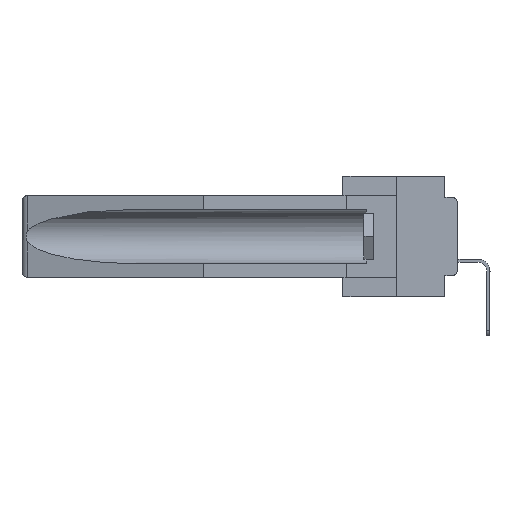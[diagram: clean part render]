
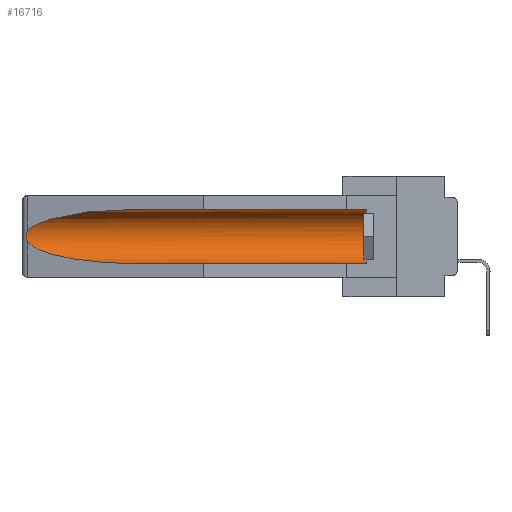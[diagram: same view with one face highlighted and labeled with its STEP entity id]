
A CAD part, left-side view. The second image highlights one B-rep face of the part: STEP entity #16716.
In plain terms, the highlighted cylindrical face has radius 2.857 mm (diameter 5.715 mm), a partial arc.
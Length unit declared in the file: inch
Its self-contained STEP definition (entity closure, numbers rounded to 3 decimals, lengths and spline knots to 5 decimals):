
#105 = CARTESIAN_POINT ( 'NONE',  ( 0.155, -0.30754, -0.059 ) ) ;
#718 = CARTESIAN_POINT ( 'NONE',  ( 0.26537, 1.52718, -0.14972 ) ) ;
#1028 = CARTESIAN_POINT ( 'NONE',  ( 0.155, -0.30754, -0.1715 ) ) ;
#1640 = ORIENTED_EDGE ( 'NONE', *, *, #16192, .T. ) ;
#2006 = CARTESIAN_POINT ( 'NONE',  ( 0.155, 1.07973, -0.059 ) ) ;
#2267 = CARTESIAN_POINT ( 'NONE',  ( 0.155, 1.07973, -0.284 ) ) ;
#2956 = VERTEX_POINT ( 'NONE', #7251 ) ;
#3813 = VERTEX_POINT ( 'NONE', #2006 ) ;
#4181 = CARTESIAN_POINT ( 'NONE',  ( 0.155, 0.126, -0.059 ) ) ;
#4958 = CARTESIAN_POINT ( 'NONE',  ( 0.26654, 1.53092, -0.15636 ) ) ;
#5268 = EDGE_LOOP ( 'NONE', ( #12434, #22318, #27496, #17590, #1640, #22767 ) ) ;
#5561 = CYLINDRICAL_SURFACE ( 'NONE', #6483, 0.1125 ) ;
#6483 = AXIS2_PLACEMENT_3D ( 'NONE', #1028, #25777, #22662 ) ;
#7251 = CARTESIAN_POINT ( 'NONE',  ( 0.26537, 1.52718, -0.19328 ) ) ;
#7701 = CARTESIAN_POINT ( 'NONE',  ( 0.2675, 1.53308, -0.17534 ) ) ;
#8160 = B_SPLINE_CURVE_WITH_KNOTS ( 'NONE', 3,
 ( #27314, #27443, #4958, #19149, #24191, #7701, #13264, #26968, #32794, #10482 ),
 .UNSPECIFIED., .F., .F.,
 ( 4, 2, 2, 2, 4 ),
 ( 0., 0.00029, 0.00058, 0.00087, 0.00117 ),
 .UNSPECIFIED. ) ;
#8380 = VERTEX_POINT ( 'NONE', #17113 ) ;
#10026 = VERTEX_POINT ( 'NONE', #23471 ) ;
#10482 = CARTESIAN_POINT ( 'NONE',  ( 0.26537, 1.52718, -0.19328 ) ) ;
#10791 = EDGE_CURVE ( 'NONE', #2956, #8380, #33728, .T. ) ;
#12370 = DIRECTION ( 'NONE',  ( 0., -1., 0. ) ) ;
#12434 = ORIENTED_EDGE ( 'NONE', *, *, #25221, .T. ) ;
#12537 = VECTOR ( 'NONE', #16839, 39.37008 ) ;
#13201 = CARTESIAN_POINT ( 'NONE',  ( 0.21114, 1.30732, -0.284 ) ) ;
#13264 = CARTESIAN_POINT ( 'NONE',  ( 0.2673, 1.53269, -0.17917 ) ) ;
#13552 = CARTESIAN_POINT ( 'NONE',  ( 0.26537, 1.52718, -0.19328 ) ) ;
#15893 = EDGE_CURVE ( 'NONE', #18064, #3813, #24154, .T. ) ;
#15982 = CARTESIAN_POINT ( 'NONE',  ( 0.155, -0.30754, -0.284 ) ) ;
#16192 = EDGE_CURVE ( 'NONE', #10026, #18064, #18959, .T. ) ;
#16415 = LINE ( 'NONE', #15982, #34472 ) ;
#16716 = ADVANCED_FACE ( 'NONE', ( #32641 ), #5561, .F. ) ;
#16839 = DIRECTION ( 'NONE',  ( 0., 1., 0. ) ) ;
#17113 = CARTESIAN_POINT ( 'NONE',  ( 0.155, 1.07973, -0.284 ) ) ;
#17590 = ORIENTED_EDGE ( 'NONE', *, *, #20968, .F. ) ;
#18064 = VERTEX_POINT ( 'NONE', #4181 ) ;
#18959 = CIRCLE ( 'NONE', #26274, 0.1125 ) ;
#19149 = CARTESIAN_POINT ( 'NONE',  ( 0.2673, 1.5327, -0.16383 ) ) ;
#20650 = DIRECTION ( 'NONE',  ( 0., 0., 1. ) ) ;
#20968 = EDGE_CURVE ( 'NONE', #10026, #8380, #16415, .T. ) ;
#22318 = ORIENTED_EDGE ( 'NONE', *, *, #25364, .T. ) ;
#22662 = DIRECTION ( 'NONE',  ( 0., 0., 1. ) ) ;
#22767 = ORIENTED_EDGE ( 'NONE', *, *, #15893, .T. ) ;
#23471 = CARTESIAN_POINT ( 'NONE',  ( 0.155, 0.126, -0.284 ) ) ;
#23950 = CARTESIAN_POINT ( 'NONE',  ( 0.21114, 1.30732, -0.059 ) ) ;
#24154 = LINE ( 'NONE', #105, #12537 ) ;
#24191 = CARTESIAN_POINT ( 'NONE',  ( 0.2675, 1.53308, -0.16763 ) ) ;
#25221 = EDGE_CURVE ( 'NONE', #3813, #33127, #32180, .T. ) ;
#25364 = EDGE_CURVE ( 'NONE', #33127, #2956, #8160, .T. ) ;
#25777 = DIRECTION ( 'NONE',  ( 0., 1., 0. ) ) ;
#26274 = AXIS2_PLACEMENT_3D ( 'NONE', #28822, #12370, #20650 ) ;
#26742 = CARTESIAN_POINT ( 'NONE',  ( 0.25451, 1.48313, -0.09465 ) ) ;
#26968 = CARTESIAN_POINT ( 'NONE',  ( 0.26655, 1.53094, -0.18657 ) ) ;
#27025 = CARTESIAN_POINT ( 'NONE',  ( 0.25451, 1.48313, -0.24835 ) ) ;
#27314 = CARTESIAN_POINT ( 'NONE',  ( 0.26537, 1.52718, -0.14972 ) ) ;
#27443 = CARTESIAN_POINT ( 'NONE',  ( 0.26597, 1.52961, -0.15275 ) ) ;
#27496 = ORIENTED_EDGE ( 'NONE', *, *, #10791, .T. ) ;
#28822 = CARTESIAN_POINT ( 'NONE',  ( 0.155, 0.126, -0.1715 ) ) ;
#29781 = DIRECTION ( 'NONE',  ( 0., 1., 0. ) ) ;
#31985 = CARTESIAN_POINT ( 'NONE',  ( 0.155, 1.07973, -0.059 ) ) ;
#32180 =( BOUNDED_CURVE ( )  B_SPLINE_CURVE ( 3, ( #31985, #23950, #26742, #35119 ),
 .UNSPECIFIED., .F., .T. ) 
 B_SPLINE_CURVE_WITH_KNOTS ( ( 4, 4 ),
 ( 4.71239, 6.08839 ),
 .UNSPECIFIED. ) 
 CURVE ( )  GEOMETRIC_REPRESENTATION_ITEM ( )  RATIONAL_B_SPLINE_CURVE ( ( 1., 0.848, 0.848, 1. ) ) 
 REPRESENTATION_ITEM ( '' )  );
#32641 = FACE_OUTER_BOUND ( 'NONE', #5268, .T. ) ;
#32794 = CARTESIAN_POINT ( 'NONE',  ( 0.26597, 1.5296, -0.19026 ) ) ;
#33127 = VERTEX_POINT ( 'NONE', #718 ) ;
#33728 =( BOUNDED_CURVE ( )  B_SPLINE_CURVE ( 3, ( #13552, #27025, #13201, #2267 ),
 .UNSPECIFIED., .F., .F. ) 
 B_SPLINE_CURVE_WITH_KNOTS ( ( 4, 4 ),
 ( 0.1948, 1.5708 ),
 .UNSPECIFIED. ) 
 CURVE ( )  GEOMETRIC_REPRESENTATION_ITEM ( )  RATIONAL_B_SPLINE_CURVE ( ( 1., 0.848, 0.848, 1. ) ) 
 REPRESENTATION_ITEM ( '' )  );
#34472 = VECTOR ( 'NONE', #29781, 39.37008 ) ;
#35119 = CARTESIAN_POINT ( 'NONE',  ( 0.26537, 1.52718, -0.14972 ) ) ;
